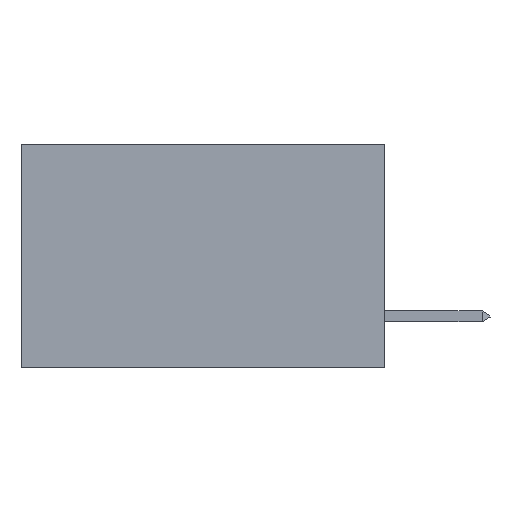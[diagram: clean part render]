
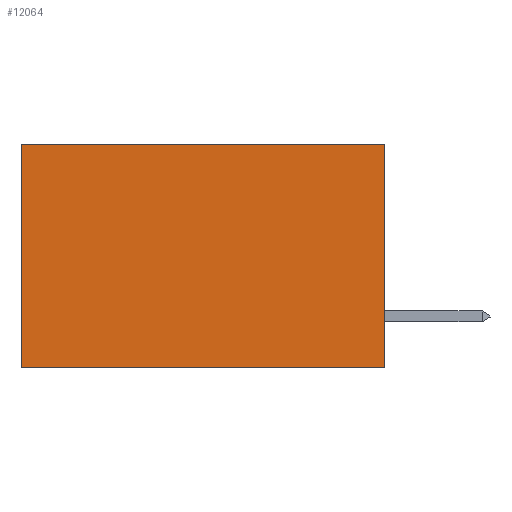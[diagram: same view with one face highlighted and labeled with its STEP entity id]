
A CAD part, left-side view. The second image highlights one B-rep face of the part: STEP entity #12064.
In plain terms, the highlighted planar face has unit normal (-1, 0, 0).
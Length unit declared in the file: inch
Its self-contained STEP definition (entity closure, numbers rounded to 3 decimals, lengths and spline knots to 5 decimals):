
#663 = DIRECTION ( 'NONE',  ( 0., 1., 0. ) ) ;
#901 = VERTEX_POINT ( 'NONE', #10573 ) ;
#1296 = VERTEX_POINT ( 'NONE', #4010 ) ;
#1795 = VECTOR ( 'NONE', #4279, 39.37008 ) ;
#1963 = VECTOR ( 'NONE', #11483, 39.37008 ) ;
#2275 = EDGE_CURVE ( 'NONE', #5083, #10069, #13736, .T. ) ;
#2654 = CARTESIAN_POINT ( 'NONE',  ( 0.2875, 0., 0. ) ) ;
#3194 = CARTESIAN_POINT ( 'NONE',  ( 0.2875, 0., 0. ) ) ;
#3737 = VECTOR ( 'NONE', #663, 39.37008 ) ;
#4010 = CARTESIAN_POINT ( 'NONE',  ( 0.2875, 0.6, -0.37 ) ) ;
#4279 = DIRECTION ( 'NONE',  ( 0., 0., -1. ) ) ;
#5083 = VERTEX_POINT ( 'NONE', #2654 ) ;
#5479 = CARTESIAN_POINT ( 'NONE',  ( 0.2875, 0., 0. ) ) ;
#6245 = DIRECTION ( 'NONE',  ( 1., 0., 0. ) ) ;
#6519 = EDGE_LOOP ( 'NONE', ( #13498, #8987, #14068, #6600 ) ) ;
#6600 = ORIENTED_EDGE ( 'NONE', *, *, #17755, .T. ) ;
#6657 = CARTESIAN_POINT ( 'NONE',  ( 0.2875, 0., -0.37 ) ) ;
#7086 = AXIS2_PLACEMENT_3D ( 'NONE', #3194, #6245, #16550 ) ;
#7410 = CARTESIAN_POINT ( 'NONE',  ( 0.2875, 0., 0. ) ) ;
#7772 = LINE ( 'NONE', #6657, #3737 ) ;
#7917 = FACE_OUTER_BOUND ( 'NONE', #6519, .T. ) ;
#8987 = ORIENTED_EDGE ( 'NONE', *, *, #9122, .F. ) ;
#9122 = EDGE_CURVE ( 'NONE', #10069, #1296, #7772, .T. ) ;
#10069 = VERTEX_POINT ( 'NONE', #10353 ) ;
#10353 = CARTESIAN_POINT ( 'NONE',  ( 0.2875, 0., -0.37 ) ) ;
#10573 = CARTESIAN_POINT ( 'NONE',  ( 0.2875, 0.6, 0. ) ) ;
#10643 = PLANE ( 'NONE',  #7086 ) ;
#11462 = VECTOR ( 'NONE', #14376, 39.37008 ) ;
#11483 = DIRECTION ( 'NONE',  ( 0., 0., -1. ) ) ;
#12064 = ADVANCED_FACE ( 'NONE', ( #7917 ), #10643, .F. ) ;
#13050 = EDGE_CURVE ( 'NONE', #901, #1296, #17678, .T. ) ;
#13498 = ORIENTED_EDGE ( 'NONE', *, *, #13050, .T. ) ;
#13736 = LINE ( 'NONE', #7410, #1795 ) ;
#14068 = ORIENTED_EDGE ( 'NONE', *, *, #2275, .F. ) ;
#14376 = DIRECTION ( 'NONE',  ( 0., 1., 0. ) ) ;
#14961 = LINE ( 'NONE', #5479, #11462 ) ;
#16550 = DIRECTION ( 'NONE',  ( 0., 0., -1. ) ) ;
#17678 = LINE ( 'NONE', #18685, #1963 ) ;
#17755 = EDGE_CURVE ( 'NONE', #5083, #901, #14961, .T. ) ;
#18685 = CARTESIAN_POINT ( 'NONE',  ( 0.2875, 0.6, 0. ) ) ;
